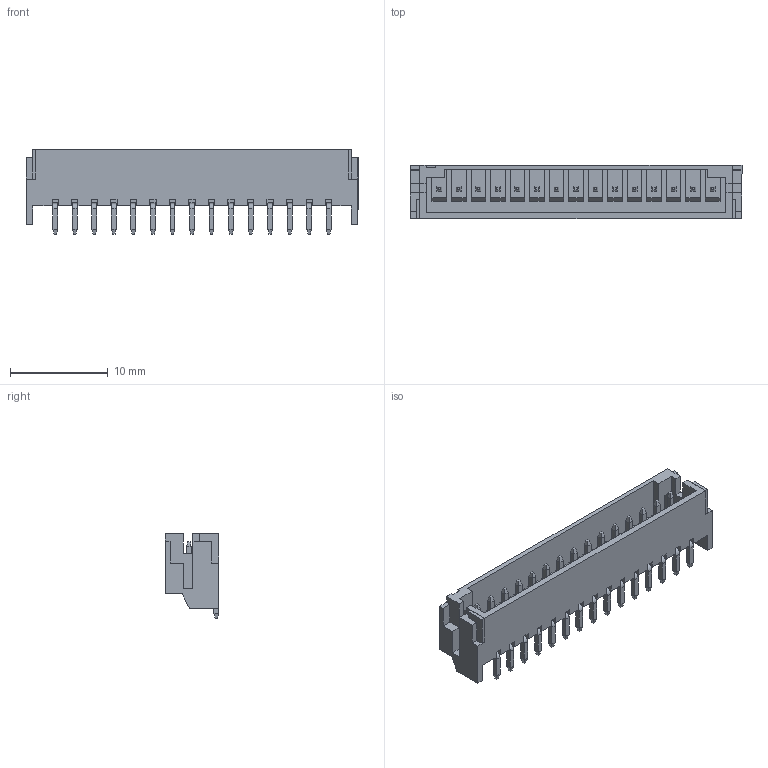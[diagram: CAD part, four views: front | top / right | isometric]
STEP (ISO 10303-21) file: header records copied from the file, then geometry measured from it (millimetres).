
FILE_DESCRIPTION (( 'STEP AP203' ), '1' );
FILE_NAME ('140-515-417-060.STEP', '2020-03-31T20:26:10', ( '' ), ( '' ), 'SwSTEP 2.0', 'SolidWorks 2016', '' );
FILE_SCHEMA (( 'CONFIG_CONTROL_DESIGN' ));
Length unit declared in the file: millimetre
Products named in the file (4): RA SMT Contact; RA SMT Pad; RA SMT Housing_515; 140-515-417-060
Assembly tree (18 placements, depth 2):
  140-515-417-060
    RA SMT Housing_515
    RA SMT Contact  x15
    RA SMT Pad  x2
Bounding box: 34 x 5.5 x 8.65 mm (x, y, z)
Volume: 443.6 mm3; surface area: 1701.3 mm2
Topology: 18 solids, 18 shells, 770 faces, 1852 edges, 1114 vertices
Faces by surface type: plane 710, cylinder 60
Entity records: 12046 total; most frequent: CARTESIAN_POINT 2023, ORIENTED_EDGE 2000, DIRECTION 1738, EDGE_CURVE 1000, LINE 992, VECTOR 992, VERTEX_POINT 658, EDGE_LOOP 374
